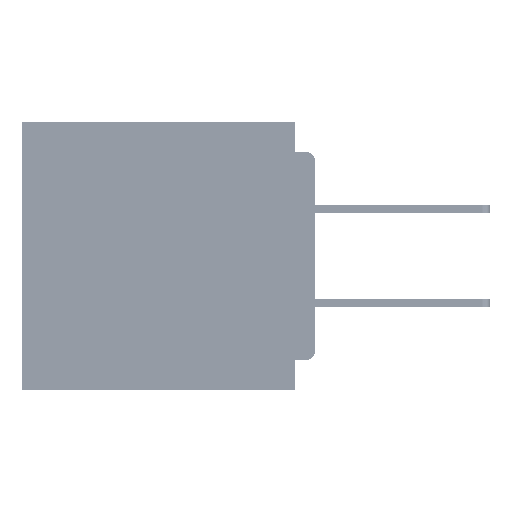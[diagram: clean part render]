
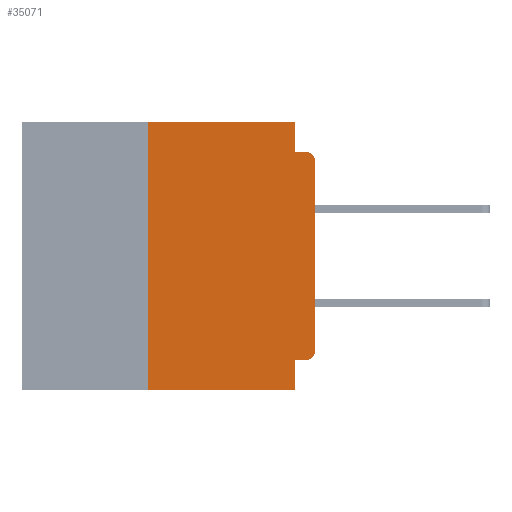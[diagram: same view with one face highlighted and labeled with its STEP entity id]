
A CAD part, left-side view. The second image highlights one B-rep face of the part: STEP entity #35071.
In plain terms, the highlighted planar face has unit normal (-1, 0, 0).
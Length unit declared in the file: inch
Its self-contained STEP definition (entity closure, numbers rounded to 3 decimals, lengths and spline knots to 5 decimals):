
#58 = CARTESIAN_POINT ( 'NONE',  ( 0., 0.437, 0. ) ) ;
#967 = ORIENTED_EDGE ( 'NONE', *, *, #7588, .T. ) ;
#1883 = CARTESIAN_POINT ( 'NONE',  ( 0., 0.25, -0.4 ) ) ;
#1891 = VECTOR ( 'NONE', #14150, 39.37008 ) ;
#2190 = ORIENTED_EDGE ( 'NONE', *, *, #33333, .F. ) ;
#2573 = CIRCLE ( 'NONE', #7951, 0.015 ) ;
#3601 = LINE ( 'NONE', #57644, #1891 ) ;
#3871 = DIRECTION ( 'NONE',  ( 0., -1., 0. ) ) ;
#4924 = CARTESIAN_POINT ( 'NONE',  ( 0., 0.031, 0. ) ) ;
#5489 = DIRECTION ( 'NONE',  ( 0., 0., -1. ) ) ;
#6491 = CARTESIAN_POINT ( 'NONE',  ( 0., 0., -0.34 ) ) ;
#7125 = LINE ( 'NONE', #35400, #18170 ) ;
#7588 = EDGE_CURVE ( 'NONE', #54269, #49199, #47830, .T. ) ;
#7872 = VERTEX_POINT ( 'NONE', #69853 ) ;
#7951 = AXIS2_PLACEMENT_3D ( 'NONE', #45555, #13047, #51045 ) ;
#8103 = CARTESIAN_POINT ( 'NONE',  ( 0., 0.25, 0. ) ) ;
#9374 = VECTOR ( 'NONE', #53881, 39.37008 ) ;
#11767 = LINE ( 'NONE', #58032, #22783 ) ;
#12128 = LINE ( 'NONE', #69212, #68167 ) ;
#12180 = ORIENTED_EDGE ( 'NONE', *, *, #16208, .F. ) ;
#12285 = ORIENTED_EDGE ( 'NONE', *, *, #38611, .F. ) ;
#13047 = DIRECTION ( 'NONE',  ( -1., 0., 0. ) ) ;
#13660 = CARTESIAN_POINT ( 'NONE',  ( 0., 0., 0. ) ) ;
#14058 = LINE ( 'NONE', #63064, #42905 ) ;
#14150 = DIRECTION ( 'NONE',  ( 0., 0., 1. ) ) ;
#16208 = EDGE_CURVE ( 'NONE', #36504, #23930, #7125, .T. ) ;
#16449 = CARTESIAN_POINT ( 'NONE',  ( 0., 0.031, -0.4 ) ) ;
#17074 = ORIENTED_EDGE ( 'NONE', *, *, #17782, .F. ) ;
#17414 = EDGE_LOOP ( 'NONE', ( #967, #35831, #12285, #39697, #2190, #17074, #53575, #24733, #12180, #23162 ) ) ;
#17476 = DIRECTION ( 'NONE',  ( -1., 0., 0. ) ) ;
#17782 = EDGE_CURVE ( 'NONE', #35287, #64418, #3601, .T. ) ;
#18170 = VECTOR ( 'NONE', #40834, 39.37008 ) ;
#18882 = EDGE_CURVE ( 'NONE', #49199, #48429, #2573, .T. ) ;
#19749 = CARTESIAN_POINT ( 'NONE',  ( 0., 0.031, 0. ) ) ;
#22783 = VECTOR ( 'NONE', #41565, 39.37008 ) ;
#23162 = ORIENTED_EDGE ( 'NONE', *, *, #55864, .T. ) ;
#23290 = LINE ( 'NONE', #41822, #66642 ) ;
#23773 = LINE ( 'NONE', #4924, #9374 ) ;
#23930 = VERTEX_POINT ( 'NONE', #36013 ) ;
#24733 = ORIENTED_EDGE ( 'NONE', *, *, #59335, .F. ) ;
#25999 = DIRECTION ( 'NONE',  ( 0., -1., 0. ) ) ;
#27181 = EDGE_CURVE ( 'NONE', #34844, #7872, #23773, .T. ) ;
#27288 = CIRCLE ( 'NONE', #49961, 0.015 ) ;
#30528 = DIRECTION ( 'NONE',  ( 0., -1., 0. ) ) ;
#31703 = CARTESIAN_POINT ( 'NONE',  ( 0., 0., -0.06 ) ) ;
#32540 = PLANE ( 'NONE',  #33897 ) ;
#33333 = EDGE_CURVE ( 'NONE', #64418, #34844, #12128, .T. ) ;
#33897 = AXIS2_PLACEMENT_3D ( 'NONE', #58, #37991, #5489 ) ;
#34844 = VERTEX_POINT ( 'NONE', #19749 ) ;
#35045 = VECTOR ( 'NONE', #51650, 39.37008 ) ;
#35071 = ADVANCED_FACE ( 'NONE', ( #69618 ), #32540, .F. ) ;
#35287 = VERTEX_POINT ( 'NONE', #1883 ) ;
#35400 = CARTESIAN_POINT ( 'NONE',  ( 0., 0., -0.355 ) ) ;
#35831 = ORIENTED_EDGE ( 'NONE', *, *, #18882, .T. ) ;
#36013 = CARTESIAN_POINT ( 'NONE',  ( 0., 0.031, -0.355 ) ) ;
#36504 = VERTEX_POINT ( 'NONE', #46150 ) ;
#37991 = DIRECTION ( 'NONE',  ( 1., 0., 0. ) ) ;
#38611 = EDGE_CURVE ( 'NONE', #7872, #48429, #23290, .T. ) ;
#39697 = ORIENTED_EDGE ( 'NONE', *, *, #27181, .F. ) ;
#40834 = DIRECTION ( 'NONE',  ( 0., 1., 0. ) ) ;
#41565 = DIRECTION ( 'NONE',  ( 0., 0., -1. ) ) ;
#41822 = CARTESIAN_POINT ( 'NONE',  ( 0., 0., -0.045 ) ) ;
#42905 = VECTOR ( 'NONE', #30528, 39.37008 ) ;
#45555 = CARTESIAN_POINT ( 'NONE',  ( 0., 0.015, -0.06 ) ) ;
#46150 = CARTESIAN_POINT ( 'NONE',  ( 0., 0.015, -0.355 ) ) ;
#47572 = VERTEX_POINT ( 'NONE', #16449 ) ;
#47830 = LINE ( 'NONE', #13660, #35045 ) ;
#48429 = VERTEX_POINT ( 'NONE', #50272 ) ;
#49199 = VERTEX_POINT ( 'NONE', #31703 ) ;
#49961 = AXIS2_PLACEMENT_3D ( 'NONE', #50002, #17476, #55510 ) ;
#50002 = CARTESIAN_POINT ( 'NONE',  ( 0., 0.015, -0.34 ) ) ;
#50272 = CARTESIAN_POINT ( 'NONE',  ( 0., 0.015, -0.045 ) ) ;
#51045 = DIRECTION ( 'NONE',  ( 0., 0., -1. ) ) ;
#51650 = DIRECTION ( 'NONE',  ( 0., 0., 1. ) ) ;
#53575 = ORIENTED_EDGE ( 'NONE', *, *, #53815, .T. ) ;
#53815 = EDGE_CURVE ( 'NONE', #35287, #47572, #14058, .T. ) ;
#53881 = DIRECTION ( 'NONE',  ( 0., 0., -1. ) ) ;
#54269 = VERTEX_POINT ( 'NONE', #6491 ) ;
#55510 = DIRECTION ( 'NONE',  ( 0., 0., -1. ) ) ;
#55864 = EDGE_CURVE ( 'NONE', #36504, #54269, #27288, .T. ) ;
#57644 = CARTESIAN_POINT ( 'NONE',  ( 0., 0.25, -0.4 ) ) ;
#58032 = CARTESIAN_POINT ( 'NONE',  ( 0., 0.031, -0.4 ) ) ;
#59335 = EDGE_CURVE ( 'NONE', #23930, #47572, #11767, .T. ) ;
#63064 = CARTESIAN_POINT ( 'NONE',  ( 0., 0.437, -0.4 ) ) ;
#64418 = VERTEX_POINT ( 'NONE', #8103 ) ;
#66642 = VECTOR ( 'NONE', #3871, 39.37008 ) ;
#68167 = VECTOR ( 'NONE', #25999, 39.37008 ) ;
#69212 = CARTESIAN_POINT ( 'NONE',  ( 0., 0.437, 0. ) ) ;
#69618 = FACE_OUTER_BOUND ( 'NONE', #17414, .T. ) ;
#69853 = CARTESIAN_POINT ( 'NONE',  ( 0., 0.031, -0.045 ) ) ;
